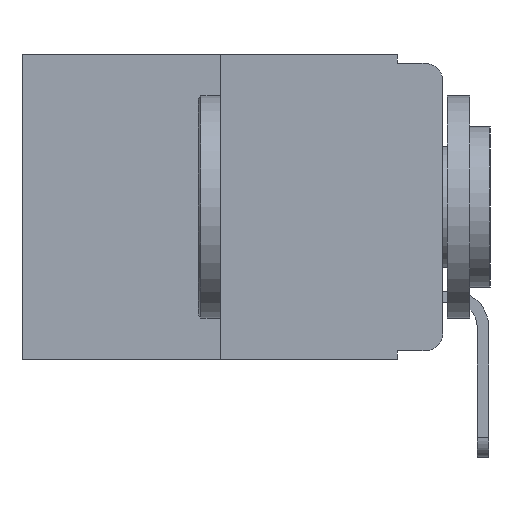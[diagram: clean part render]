
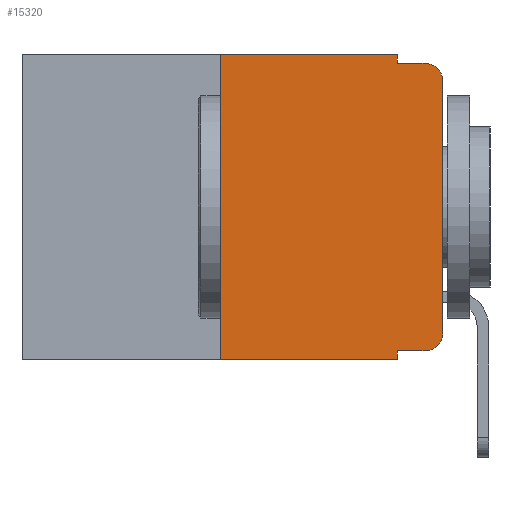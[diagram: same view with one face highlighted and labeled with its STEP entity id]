
A CAD part, left-side view. The second image highlights one B-rep face of the part: STEP entity #15320.
In plain terms, the highlighted planar face has unit normal (-1, 0, 0).
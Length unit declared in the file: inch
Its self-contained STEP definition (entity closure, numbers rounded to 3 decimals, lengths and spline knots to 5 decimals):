
#401 = DIRECTION ( 'NONE',  ( 0., -1., 0. ) ) ;
#435 = VERTEX_POINT ( 'NONE', #8352 ) ;
#767 = LINE ( 'NONE', #2125, #6539 ) ;
#775 = VECTOR ( 'NONE', #13788, 39.37008 ) ;
#789 = EDGE_CURVE ( 'NONE', #5891, #435, #13975, .T. ) ;
#905 = VECTOR ( 'NONE', #6350, 39.37008 ) ;
#1240 = VECTOR ( 'NONE', #6064, 39.37008 ) ;
#1405 = DIRECTION ( 'NONE',  ( 0., 0., -1. ) ) ;
#1685 = LINE ( 'NONE', #9150, #15025 ) ;
#1747 = DIRECTION ( 'NONE',  ( 0., 0., -1. ) ) ;
#1787 = LINE ( 'NONE', #6679, #14606 ) ;
#1865 = CARTESIAN_POINT ( 'NONE',  ( 0., 0.25, -0.343 ) ) ;
#2025 = ORIENTED_EDGE ( 'NONE', *, *, #10539, .T. ) ;
#2125 = CARTESIAN_POINT ( 'NONE',  ( 0., 0.051, -0.333 ) ) ;
#2140 = CARTESIAN_POINT ( 'NONE',  ( 0., 0.051, -0.01 ) ) ;
#2611 = PLANE ( 'NONE',  #5115 ) ;
#2933 = ORIENTED_EDGE ( 'NONE', *, *, #14167, .T. ) ;
#2950 = ORIENTED_EDGE ( 'NONE', *, *, #15285, .F. ) ;
#3596 = LINE ( 'NONE', #8503, #13491 ) ;
#3651 = CARTESIAN_POINT ( 'NONE',  ( 0., 0.02, -0.01 ) ) ;
#3953 = CARTESIAN_POINT ( 'NONE',  ( 0., 0., -0.03 ) ) ;
#3998 = VERTEX_POINT ( 'NONE', #7534 ) ;
#4041 = CARTESIAN_POINT ( 'NONE',  ( 0., 0.473, 0. ) ) ;
#4207 = ORIENTED_EDGE ( 'NONE', *, *, #15167, .F. ) ;
#4445 = CARTESIAN_POINT ( 'NONE',  ( 0., 0.02, -0.333 ) ) ;
#4678 = CARTESIAN_POINT ( 'NONE',  ( 0., 0., -0.313 ) ) ;
#5051 = CARTESIAN_POINT ( 'NONE',  ( 0., 0., 0. ) ) ;
#5079 = CIRCLE ( 'NONE', #14087, 0.02 ) ;
#5115 = AXIS2_PLACEMENT_3D ( 'NONE', #4041, #6217, #1405 ) ;
#5399 = EDGE_CURVE ( 'NONE', #9087, #5582, #10387, .T. ) ;
#5582 = VERTEX_POINT ( 'NONE', #3651 ) ;
#5649 = ORIENTED_EDGE ( 'NONE', *, *, #15884, .F. ) ;
#5891 = VERTEX_POINT ( 'NONE', #13285 ) ;
#6028 = EDGE_CURVE ( 'NONE', #10465, #9087, #11320, .T. ) ;
#6064 = DIRECTION ( 'NONE',  ( 0., 0., 1. ) ) ;
#6217 = DIRECTION ( 'NONE',  ( 1., 0., 0. ) ) ;
#6350 = DIRECTION ( 'NONE',  ( 0., 0., 1. ) ) ;
#6459 = FACE_OUTER_BOUND ( 'NONE', #10376, .T. ) ;
#6503 = EDGE_CURVE ( 'NONE', #15696, #3998, #1685, .T. ) ;
#6539 = VECTOR ( 'NONE', #10555, 39.37008 ) ;
#6679 = CARTESIAN_POINT ( 'NONE',  ( 0., 0.051, -0.01 ) ) ;
#6830 = EDGE_CURVE ( 'NONE', #7945, #435, #3596, .T. ) ;
#7238 = ORIENTED_EDGE ( 'NONE', *, *, #6830, .T. ) ;
#7534 = CARTESIAN_POINT ( 'NONE',  ( 0., 0.051, 0. ) ) ;
#7553 = ORIENTED_EDGE ( 'NONE', *, *, #789, .F. ) ;
#7673 = CARTESIAN_POINT ( 'NONE',  ( 0., 0.051, 0. ) ) ;
#7712 = ORIENTED_EDGE ( 'NONE', *, *, #5399, .T. ) ;
#7815 = ORIENTED_EDGE ( 'NONE', *, *, #6503, .F. ) ;
#7945 = VERTEX_POINT ( 'NONE', #1865 ) ;
#8094 = DIRECTION ( 'NONE',  ( -1., 0., 0. ) ) ;
#8352 = CARTESIAN_POINT ( 'NONE',  ( 0., 0.051, -0.343 ) ) ;
#8503 = CARTESIAN_POINT ( 'NONE',  ( 0., 0.473, -0.343 ) ) ;
#9087 = VERTEX_POINT ( 'NONE', #3953 ) ;
#9150 = CARTESIAN_POINT ( 'NONE',  ( 0., 0.473, 0. ) ) ;
#9679 = AXIS2_PLACEMENT_3D ( 'NONE', #15335, #8094, #1747 ) ;
#10190 = CARTESIAN_POINT ( 'NONE',  ( 0., 0.02, -0.313 ) ) ;
#10344 = DIRECTION ( 'NONE',  ( -1., 0., 0. ) ) ;
#10376 = EDGE_LOOP ( 'NONE', ( #12900, #7712, #5649, #2950, #7815, #4207, #7238, #7553, #2025, #2933 ) ) ;
#10387 = CIRCLE ( 'NONE', #9679, 0.02 ) ;
#10434 = VERTEX_POINT ( 'NONE', #4445 ) ;
#10465 = VERTEX_POINT ( 'NONE', #4678 ) ;
#10539 = EDGE_CURVE ( 'NONE', #5891, #10434, #767, .T. ) ;
#10555 = DIRECTION ( 'NONE',  ( 0., -1., 0. ) ) ;
#10807 = LINE ( 'NONE', #13376, #1240 ) ;
#11117 = LINE ( 'NONE', #7673, #775 ) ;
#11222 = CARTESIAN_POINT ( 'NONE',  ( 0., 0.051, 0. ) ) ;
#11303 = DIRECTION ( 'NONE',  ( 0., 0., -1. ) ) ;
#11320 = LINE ( 'NONE', #5051, #905 ) ;
#11575 = DIRECTION ( 'NONE',  ( 0., -1., 0. ) ) ;
#11874 = VECTOR ( 'NONE', #11303, 39.37008 ) ;
#12470 = CARTESIAN_POINT ( 'NONE',  ( 0., 0.25, 0. ) ) ;
#12900 = ORIENTED_EDGE ( 'NONE', *, *, #6028, .T. ) ;
#13285 = CARTESIAN_POINT ( 'NONE',  ( 0., 0.051, -0.333 ) ) ;
#13376 = CARTESIAN_POINT ( 'NONE',  ( 0., 0.25, 0. ) ) ;
#13400 = DIRECTION ( 'NONE',  ( 0., -1., 0. ) ) ;
#13491 = VECTOR ( 'NONE', #13400, 39.37008 ) ;
#13788 = DIRECTION ( 'NONE',  ( 0., 0., -1. ) ) ;
#13975 = LINE ( 'NONE', #11222, #11874 ) ;
#14087 = AXIS2_PLACEMENT_3D ( 'NONE', #10190, #10344, #15104 ) ;
#14167 = EDGE_CURVE ( 'NONE', #10434, #10465, #5079, .T. ) ;
#14606 = VECTOR ( 'NONE', #11575, 39.37008 ) ;
#15025 = VECTOR ( 'NONE', #401, 39.37008 ) ;
#15090 = VERTEX_POINT ( 'NONE', #2140 ) ;
#15104 = DIRECTION ( 'NONE',  ( 0., 0., -1. ) ) ;
#15167 = EDGE_CURVE ( 'NONE', #7945, #15696, #10807, .T. ) ;
#15285 = EDGE_CURVE ( 'NONE', #3998, #15090, #11117, .T. ) ;
#15320 = ADVANCED_FACE ( 'NONE', ( #6459 ), #2611, .F. ) ;
#15335 = CARTESIAN_POINT ( 'NONE',  ( 0., 0.02, -0.03 ) ) ;
#15696 = VERTEX_POINT ( 'NONE', #12470 ) ;
#15884 = EDGE_CURVE ( 'NONE', #15090, #5582, #1787, .T. ) ;
